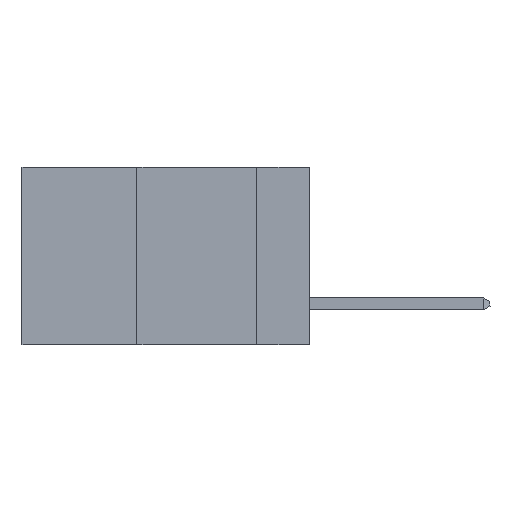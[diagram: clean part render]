
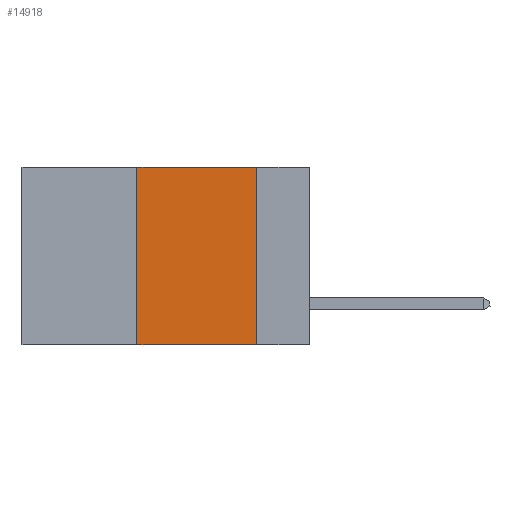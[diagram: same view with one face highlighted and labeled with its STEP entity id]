
A CAD part, left-side view. The second image highlights one B-rep face of the part: STEP entity #14918.
In plain terms, the highlighted planar face has unit normal (-1, 0, 0).
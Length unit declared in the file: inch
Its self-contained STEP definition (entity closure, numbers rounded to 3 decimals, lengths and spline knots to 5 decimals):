
#747 = ORIENTED_EDGE ( 'NONE', *, *, #15889, .F. ) ;
#1121 = EDGE_CURVE ( 'NONE', #34624, #6591, #22825, .T. ) ;
#1165 = ORIENTED_EDGE ( 'NONE', *, *, #8145, .T. ) ;
#2501 = EDGE_LOOP ( 'NONE', ( #5048, #5786, #747, #1165 ) ) ;
#3424 = VERTEX_POINT ( 'NONE', #20335 ) ;
#5048 = ORIENTED_EDGE ( 'NONE', *, *, #12598, .F. ) ;
#5610 = CARTESIAN_POINT ( 'NONE',  ( 0., 0.11, 0. ) ) ;
#5786 = ORIENTED_EDGE ( 'NONE', *, *, #1121, .F. ) ;
#6272 = LINE ( 'NONE', #7262, #27659 ) ;
#6591 = VERTEX_POINT ( 'NONE', #5610 ) ;
#6700 = DIRECTION ( 'NONE',  ( 0., -1., 0. ) ) ;
#7088 = LINE ( 'NONE', #17096, #11955 ) ;
#7262 = CARTESIAN_POINT ( 'NONE',  ( 0., 0.6, -0.37 ) ) ;
#7482 = CARTESIAN_POINT ( 'NONE',  ( 0., 0.6, 0. ) ) ;
#8145 = EDGE_CURVE ( 'NONE', #17047, #3424, #6272, .T. ) ;
#10149 = DIRECTION ( 'NONE',  ( 1., 0., 0. ) ) ;
#11955 = VECTOR ( 'NONE', #22639, 39.37008 ) ;
#12598 = EDGE_CURVE ( 'NONE', #6591, #3424, #32486, .T. ) ;
#13775 = FACE_OUTER_BOUND ( 'NONE', #2501, .T. ) ;
#14918 = ADVANCED_FACE ( 'NONE', ( #13775 ), #26780, .F. ) ;
#15889 = EDGE_CURVE ( 'NONE', #17047, #34624, #7088, .T. ) ;
#17047 = VERTEX_POINT ( 'NONE', #19705 ) ;
#17096 = CARTESIAN_POINT ( 'NONE',  ( 0., 0.36, 0. ) ) ;
#19705 = CARTESIAN_POINT ( 'NONE',  ( 0., 0.36, -0.37 ) ) ;
#20335 = CARTESIAN_POINT ( 'NONE',  ( 0., 0.11, -0.37 ) ) ;
#21131 = CARTESIAN_POINT ( 'NONE',  ( 0., 0.6, 0. ) ) ;
#21224 = DIRECTION ( 'NONE',  ( 0., -1., 0. ) ) ;
#22639 = DIRECTION ( 'NONE',  ( 0., 0., 1. ) ) ;
#22825 = LINE ( 'NONE', #7482, #29223 ) ;
#25182 = CARTESIAN_POINT ( 'NONE',  ( 0., 0.11, 0. ) ) ;
#26058 = VECTOR ( 'NONE', #33329, 39.37008 ) ;
#26780 = PLANE ( 'NONE',  #33273 ) ;
#27659 = VECTOR ( 'NONE', #21224, 39.37008 ) ;
#29223 = VECTOR ( 'NONE', #6700, 39.37008 ) ;
#29493 = DIRECTION ( 'NONE',  ( 0., 0., -1. ) ) ;
#31591 = CARTESIAN_POINT ( 'NONE',  ( 0., 0.36, 0. ) ) ;
#32486 = LINE ( 'NONE', #25182, #26058 ) ;
#33273 = AXIS2_PLACEMENT_3D ( 'NONE', #21131, #10149, #29493 ) ;
#33329 = DIRECTION ( 'NONE',  ( 0., 0., -1. ) ) ;
#34624 = VERTEX_POINT ( 'NONE', #31591 ) ;
